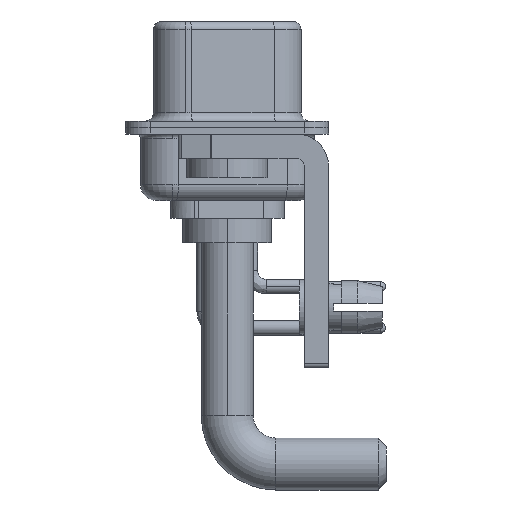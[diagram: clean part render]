
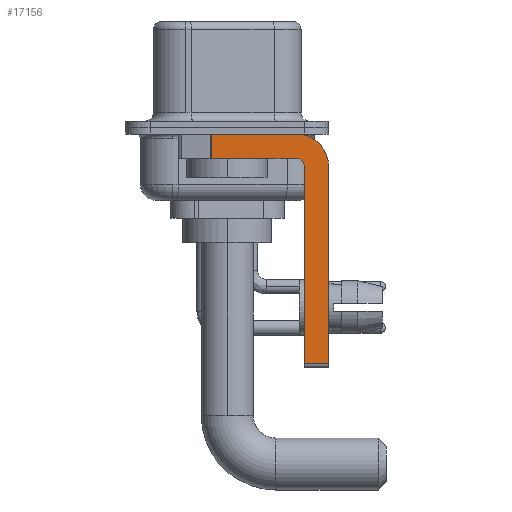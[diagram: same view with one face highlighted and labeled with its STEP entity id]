
A CAD part, left-side view. The second image highlights one B-rep face of the part: STEP entity #17156.
In plain terms, the highlighted planar face has unit normal (-1, 0, 0).
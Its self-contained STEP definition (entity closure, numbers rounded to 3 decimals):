
#583 = EDGE_CURVE ( 'NONE', #9573, #3614, #17242, .T. ) ;
#900 = DIRECTION ( 'NONE',  ( 0., 0., -1. ) ) ;
#1208 = FACE_OUTER_BOUND ( 'NONE', #23352, .T. ) ;
#1400 = CARTESIAN_POINT ( 'NONE',  ( -2.9, 3., -0.4 ) ) ;
#2311 = ORIENTED_EDGE ( 'NONE', *, *, #6843, .F. ) ;
#2678 = CARTESIAN_POINT ( 'NONE',  ( -2.9, -6.25, -2.4 ) ) ;
#3614 = VERTEX_POINT ( 'NONE', #18552 ) ;
#3746 = VECTOR ( 'NONE', #20032, 1000. ) ;
#3803 = CARTESIAN_POINT ( 'NONE',  ( -2.9, -4.75, -2.4 ) ) ;
#4312 = ORIENTED_EDGE ( 'NONE', *, *, #583, .F. ) ;
#5768 = DIRECTION ( 'NONE',  ( 0., 0., 1. ) ) ;
#5848 = CARTESIAN_POINT ( 'NONE',  ( -2.9, -4.25, -1.9 ) ) ;
#6843 = EDGE_CURVE ( 'NONE', #9166, #14986, #28814, .T. ) ;
#7172 = ORIENTED_EDGE ( 'NONE', *, *, #26212, .T. ) ;
#7386 = DIRECTION ( 'NONE',  ( 0., 0., 1. ) ) ;
#8171 = LINE ( 'NONE', #5848, #3746 ) ;
#8370 = LINE ( 'NONE', #17770, #11349 ) ;
#9166 = VERTEX_POINT ( 'NONE', #12136 ) ;
#9573 = VERTEX_POINT ( 'NONE', #2678 ) ;
#9937 = VECTOR ( 'NONE', #7386, 1000. ) ;
#10300 = CARTESIAN_POINT ( 'NONE',  ( -2.9, -4.75, -14.8 ) ) ;
#10769 = PLANE ( 'NONE',  #17277 ) ;
#10941 = DIRECTION ( 'NONE',  ( 0., 0., -1. ) ) ;
#11349 = VECTOR ( 'NONE', #27194, 1000. ) ;
#11666 = CARTESIAN_POINT ( 'NONE',  ( -2.9, 0.978, -0.4 ) ) ;
#12136 = CARTESIAN_POINT ( 'NONE',  ( -2.9, -4.75, -14.55 ) ) ;
#12222 = VECTOR ( 'NONE', #12488, 1000. ) ;
#12488 = DIRECTION ( 'NONE',  ( 0., 0., -1. ) ) ;
#12625 = ORIENTED_EDGE ( 'NONE', *, *, #28416, .F. ) ;
#12788 = DIRECTION ( 'NONE',  ( 1., 0., 0. ) ) ;
#12996 = EDGE_CURVE ( 'NONE', #25973, #29385, #8171, .T. ) ;
#13011 = VERTEX_POINT ( 'NONE', #21894 ) ;
#13229 = AXIS2_PLACEMENT_3D ( 'NONE', #17868, #22498, #10941 ) ;
#14833 = CIRCLE ( 'NONE', #22695, 0.5 ) ;
#14986 = VERTEX_POINT ( 'NONE', #3803 ) ;
#15430 = ORIENTED_EDGE ( 'NONE', *, *, #24346, .F. ) ;
#16110 = ORIENTED_EDGE ( 'NONE', *, *, #12996, .F. ) ;
#17156 = ADVANCED_FACE ( 'NONE', ( #1208 ), #10769, .F. ) ;
#17242 = LINE ( 'NONE', #17398, #12222 ) ;
#17277 = AXIS2_PLACEMENT_3D ( 'NONE', #26974, #12788, #900 ) ;
#17398 = CARTESIAN_POINT ( 'NONE',  ( -2.9, -6.25, -2.4 ) ) ;
#17770 = CARTESIAN_POINT ( 'NONE',  ( -2.9, -4.25, -14.55 ) ) ;
#17868 = CARTESIAN_POINT ( 'NONE',  ( -2.9, -4.25, -2.4 ) ) ;
#18552 = CARTESIAN_POINT ( 'NONE',  ( -2.9, -6.25, -14.55 ) ) ;
#19305 = VECTOR ( 'NONE', #27311, 1000. ) ;
#19333 = CARTESIAN_POINT ( 'NONE',  ( -2.9, -4.25, -1.9 ) ) ;
#20032 = DIRECTION ( 'NONE',  ( 0., 1., 0. ) ) ;
#21141 = VECTOR ( 'NONE', #24169, 1000. ) ;
#21604 = EDGE_CURVE ( 'NONE', #25250, #29385, #26324, .T. ) ;
#21894 = CARTESIAN_POINT ( 'NONE',  ( -2.9, -4.25, -0.4 ) ) ;
#22274 = DIRECTION ( 'NONE',  ( -1., 0., 0. ) ) ;
#22498 = DIRECTION ( 'NONE',  ( 1., 0., 0. ) ) ;
#22632 = CARTESIAN_POINT ( 'NONE',  ( -2.9, 0.978, -1.9 ) ) ;
#22695 = AXIS2_PLACEMENT_3D ( 'NONE', #24736, #22274, #5768 ) ;
#23352 = EDGE_LOOP ( 'NONE', ( #25044, #25683, #16110, #12625, #2311, #7172, #4312, #15430 ) ) ;
#24169 = DIRECTION ( 'NONE',  ( 0., 0., -1. ) ) ;
#24346 = EDGE_CURVE ( 'NONE', #13011, #9573, #26521, .T. ) ;
#24736 = CARTESIAN_POINT ( 'NONE',  ( -2.9, -4.25, -2.4 ) ) ;
#25044 = ORIENTED_EDGE ( 'NONE', *, *, #28934, .F. ) ;
#25250 = VERTEX_POINT ( 'NONE', #11666 ) ;
#25683 = ORIENTED_EDGE ( 'NONE', *, *, #21604, .T. ) ;
#25973 = VERTEX_POINT ( 'NONE', #19333 ) ;
#26212 = EDGE_CURVE ( 'NONE', #9166, #3614, #8370, .T. ) ;
#26324 = LINE ( 'NONE', #28794, #21141 ) ;
#26521 = CIRCLE ( 'NONE', #13229, 2. ) ;
#26974 = CARTESIAN_POINT ( 'NONE',  ( -2.9, -4.25, -2.4 ) ) ;
#27194 = DIRECTION ( 'NONE',  ( 0., -1., 0. ) ) ;
#27311 = DIRECTION ( 'NONE',  ( 0., -1., 0. ) ) ;
#28416 = EDGE_CURVE ( 'NONE', #14986, #25973, #14833, .T. ) ;
#28794 = CARTESIAN_POINT ( 'NONE',  ( -2.9, 0.978, -1.9 ) ) ;
#28814 = LINE ( 'NONE', #10300, #9937 ) ;
#28934 = EDGE_CURVE ( 'NONE', #25250, #13011, #29923, .T. ) ;
#29385 = VERTEX_POINT ( 'NONE', #22632 ) ;
#29923 = LINE ( 'NONE', #1400, #19305 ) ;
